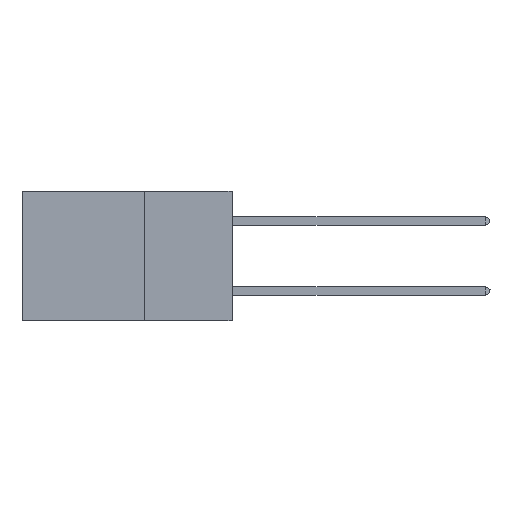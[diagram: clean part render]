
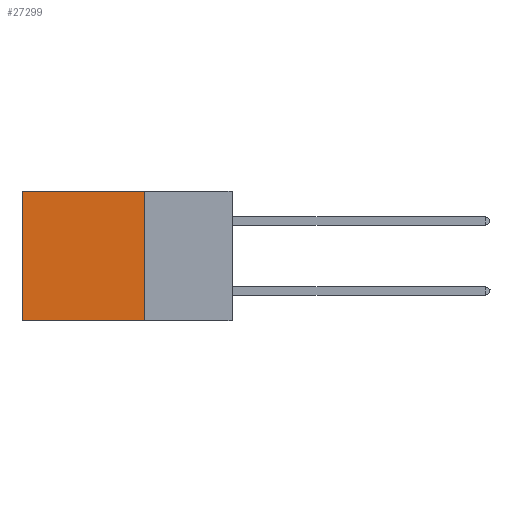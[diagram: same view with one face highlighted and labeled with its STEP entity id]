
A CAD part, left-side view. The second image highlights one B-rep face of the part: STEP entity #27299.
In plain terms, the highlighted planar face has unit normal (-1, 0, 0).
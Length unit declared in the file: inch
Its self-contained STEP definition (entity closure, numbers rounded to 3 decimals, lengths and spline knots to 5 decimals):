
#183 = ORIENTED_EDGE ( 'NONE', *, *, #23801, .T. ) ;
#668 = AXIS2_PLACEMENT_3D ( 'NONE', #16495, #12151, #27256 ) ;
#2205 = EDGE_CURVE ( 'NONE', #17666, #11138, #3876, .T. ) ;
#3784 = DIRECTION ( 'NONE',  ( 0., 1., 0. ) ) ;
#3786 = DIRECTION ( 'NONE',  ( 0., 1., 0. ) ) ;
#3876 = LINE ( 'NONE', #3913, #15119 ) ;
#3913 = CARTESIAN_POINT ( 'NONE',  ( 0.2875, 0.25, -0.37 ) ) ;
#4681 = VERTEX_POINT ( 'NONE', #9863 ) ;
#5513 = LINE ( 'NONE', #14401, #28046 ) ;
#5643 = DIRECTION ( 'NONE',  ( 0., 0., -1. ) ) ;
#6255 = ORIENTED_EDGE ( 'NONE', *, *, #2205, .F. ) ;
#8310 = EDGE_CURVE ( 'NONE', #4681, #13465, #8548, .T. ) ;
#8548 = LINE ( 'NONE', #17153, #18882 ) ;
#9863 = CARTESIAN_POINT ( 'NONE',  ( 0.2875, 0.25, 0. ) ) ;
#9909 = DIRECTION ( 'NONE',  ( 0., 0., -1. ) ) ;
#11138 = VERTEX_POINT ( 'NONE', #14061 ) ;
#12151 = DIRECTION ( 'NONE',  ( 1., 0., 0. ) ) ;
#12319 = VECTOR ( 'NONE', #5643, 39.37008 ) ;
#12596 = EDGE_CURVE ( 'NONE', #4681, #17666, #18139, .T. ) ;
#13465 = VERTEX_POINT ( 'NONE', #26247 ) ;
#13982 = ORIENTED_EDGE ( 'NONE', *, *, #12596, .F. ) ;
#14061 = CARTESIAN_POINT ( 'NONE',  ( 0.2875, 0.6, -0.37 ) ) ;
#14401 = CARTESIAN_POINT ( 'NONE',  ( 0.2875, 0.6, 0. ) ) ;
#14856 = CARTESIAN_POINT ( 'NONE',  ( 0.2875, 0.25, -0.37 ) ) ;
#15119 = VECTOR ( 'NONE', #3784, 39.37008 ) ;
#16495 = CARTESIAN_POINT ( 'NONE',  ( 0.2875, 0.25, 0. ) ) ;
#17153 = CARTESIAN_POINT ( 'NONE',  ( 0.2875, 0.25, 0. ) ) ;
#17194 = EDGE_LOOP ( 'NONE', ( #183, #6255, #13982, #22026 ) ) ;
#17666 = VERTEX_POINT ( 'NONE', #14856 ) ;
#18139 = LINE ( 'NONE', #27418, #12319 ) ;
#18882 = VECTOR ( 'NONE', #3786, 39.37008 ) ;
#22026 = ORIENTED_EDGE ( 'NONE', *, *, #8310, .T. ) ;
#22983 = PLANE ( 'NONE',  #668 ) ;
#23801 = EDGE_CURVE ( 'NONE', #13465, #11138, #5513, .T. ) ;
#26247 = CARTESIAN_POINT ( 'NONE',  ( 0.2875, 0.6, 0. ) ) ;
#27256 = DIRECTION ( 'NONE',  ( 0., 0., -1. ) ) ;
#27299 = ADVANCED_FACE ( 'NONE', ( #28159 ), #22983, .F. ) ;
#27418 = CARTESIAN_POINT ( 'NONE',  ( 0.2875, 0.25, 0. ) ) ;
#28046 = VECTOR ( 'NONE', #9909, 39.37008 ) ;
#28159 = FACE_OUTER_BOUND ( 'NONE', #17194, .T. ) ;
